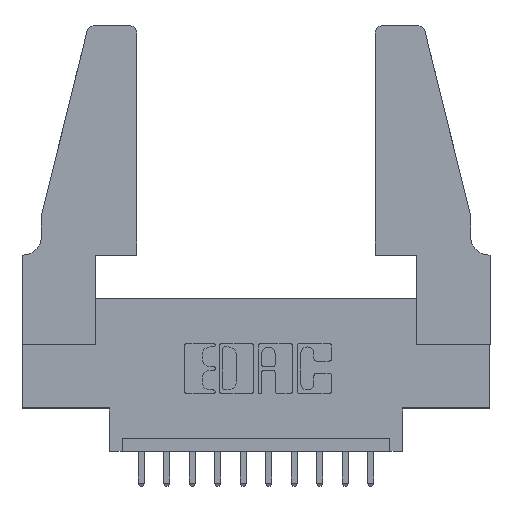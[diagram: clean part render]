
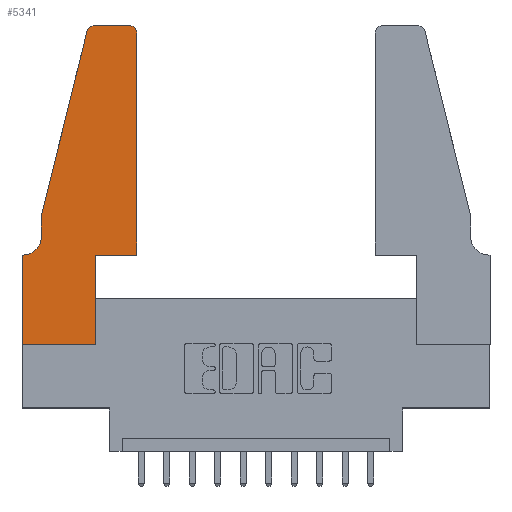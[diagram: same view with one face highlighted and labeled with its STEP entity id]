
A CAD part, top view. The second image highlights one B-rep face of the part: STEP entity #5341.
In plain terms, the highlighted planar face has unit normal (0, 0, 1).
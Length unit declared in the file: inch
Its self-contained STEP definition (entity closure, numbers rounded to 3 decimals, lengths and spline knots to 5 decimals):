
#116 = VECTOR ( 'NONE', #14130, 39.37008 ) ;
#225 = DIRECTION ( 'NONE',  ( 1., 0., 0. ) ) ;
#244 = CARTESIAN_POINT ( 'NONE',  ( 0.0755, 0.5, 0.37 ) ) ;
#553 = LINE ( 'NONE', #610, #12202 ) ;
#570 = LINE ( 'NONE', #6288, #11690 ) ;
#610 = CARTESIAN_POINT ( 'NONE',  ( 0.0755, 0.5, 0.37 ) ) ;
#613 = LINE ( 'NONE', #7789, #11924 ) ;
#923 = ORIENTED_EDGE ( 'NONE', *, *, #2108, .T. ) ;
#1114 = LINE ( 'NONE', #244, #11222 ) ;
#1170 = EDGE_CURVE ( 'NONE', #7994, #9981, #3850, .T. ) ;
#1179 = DIRECTION ( 'NONE',  ( 0., -1., 0. ) ) ;
#1343 = CARTESIAN_POINT ( 'NONE',  ( 0.2865, 0., 0.37 ) ) ;
#1762 = EDGE_CURVE ( 'NONE', #8534, #10032, #3019, .T. ) ;
#1834 = VERTEX_POINT ( 'NONE', #3236 ) ;
#1952 = ORIENTED_EDGE ( 'NONE', *, *, #5141, .T. ) ;
#1980 = CARTESIAN_POINT ( 'NONE',  ( 0.0755, 0.42, 0.37 ) ) ;
#2029 = LINE ( 'NONE', #10327, #6432 ) ;
#2077 = DIRECTION ( 'NONE',  ( 0., 0., 1. ) ) ;
#2108 = EDGE_CURVE ( 'NONE', #8501, #3767, #1114, .T. ) ;
#2338 = VERTEX_POINT ( 'NONE', #10201 ) ;
#2632 = ORIENTED_EDGE ( 'NONE', *, *, #10831, .T. ) ;
#2747 = VERTEX_POINT ( 'NONE', #6001 ) ;
#2911 = DIRECTION ( 'NONE',  ( 1., 0., 0. ) ) ;
#3019 = LINE ( 'NONE', #13044, #116 ) ;
#3236 = CARTESIAN_POINT ( 'NONE',  ( 0.4505, 0.35, 0.37 ) ) ;
#3468 = CARTESIAN_POINT ( 'NONE',  ( 0.284, 1.22, 0.37 ) ) ;
#3531 = ORIENTED_EDGE ( 'NONE', *, *, #1170, .T. ) ;
#3741 = VERTEX_POINT ( 'NONE', #11877 ) ;
#3767 = VERTEX_POINT ( 'NONE', #1980 ) ;
#3782 = EDGE_CURVE ( 'NONE', #1834, #7994, #570, .T. ) ;
#3850 = CIRCLE ( 'NONE', #4066, 0.03 ) ;
#4029 = PLANE ( 'NONE',  #7995 ) ;
#4066 = AXIS2_PLACEMENT_3D ( 'NONE', #11871, #2077, #9725 ) ;
#4172 = DIRECTION ( 'NONE',  ( 0., 1., 0. ) ) ;
#4338 = LINE ( 'NONE', #8895, #11197 ) ;
#4553 = DIRECTION ( 'NONE',  ( 0., 0., 1. ) ) ;
#4977 = CARTESIAN_POINT ( 'NONE',  ( 0.4505, 0.35, 0.37 ) ) ;
#5032 = DIRECTION ( 'NONE',  ( 0., 0., 1. ) ) ;
#5068 = DIRECTION ( 'NONE',  ( 1., 0., 0. ) ) ;
#5141 = EDGE_CURVE ( 'NONE', #2338, #7509, #2029, .T. ) ;
#5164 = CARTESIAN_POINT ( 'NONE',  ( 0.4505, 1.22, 0.37 ) ) ;
#5341 = ADVANCED_FACE ( 'NONE', ( #8469 ), #4029, .T. ) ;
#5380 = DIRECTION ( 'NONE',  ( -1., 0., 0. ) ) ;
#5451 = ORIENTED_EDGE ( 'NONE', *, *, #1762, .T. ) ;
#5857 = CIRCLE ( 'NONE', #7033, 0.03 ) ;
#6001 = CARTESIAN_POINT ( 'NONE',  ( 0.284, 1.25, 0.37 ) ) ;
#6046 = DIRECTION ( 'NONE',  ( -0.239, -0.971, 0. ) ) ;
#6053 = LINE ( 'NONE', #12047, #7571 ) ;
#6288 = CARTESIAN_POINT ( 'NONE',  ( 0.4505, 0.35, 0.37 ) ) ;
#6432 = VECTOR ( 'NONE', #8199, 39.37008 ) ;
#6453 = VECTOR ( 'NONE', #5068, 39.37008 ) ;
#6905 = EDGE_CURVE ( 'NONE', #9981, #2747, #6053, .T. ) ;
#6996 = VERTEX_POINT ( 'NONE', #13892 ) ;
#7033 = AXIS2_PLACEMENT_3D ( 'NONE', #3468, #4553, #225 ) ;
#7396 = CIRCLE ( 'NONE', #14158, 0.07 ) ;
#7486 = DIRECTION ( 'NONE',  ( -1., 0., 0. ) ) ;
#7509 = VERTEX_POINT ( 'NONE', #8205 ) ;
#7548 = EDGE_LOOP ( 'NONE', ( #11158, #7769, #9499, #923, #12934, #1952, #10941, #5451, #8616, #2632, #12844, #3531 ) ) ;
#7571 = VECTOR ( 'NONE', #5380, 39.37008 ) ;
#7769 = ORIENTED_EDGE ( 'NONE', *, *, #7992, .T. ) ;
#7789 = CARTESIAN_POINT ( 'NONE',  ( 0.2865, 0.35, 0.37 ) ) ;
#7860 = EDGE_CURVE ( 'NONE', #10032, #6996, #613, .T. ) ;
#7992 = EDGE_CURVE ( 'NONE', #2747, #3741, #5857, .T. ) ;
#7994 = VERTEX_POINT ( 'NONE', #5164 ) ;
#7995 = AXIS2_PLACEMENT_3D ( 'NONE', #11620, #5032, #2911 ) ;
#8199 = DIRECTION ( 'NONE',  ( -1., 0., 0. ) ) ;
#8205 = CARTESIAN_POINT ( 'NONE',  ( 0., 0.35, 0.37 ) ) ;
#8469 = FACE_OUTER_BOUND ( 'NONE', #7548, .T. ) ;
#8501 = VERTEX_POINT ( 'NONE', #12493 ) ;
#8534 = VERTEX_POINT ( 'NONE', #11378 ) ;
#8616 = ORIENTED_EDGE ( 'NONE', *, *, #7860, .T. ) ;
#8895 = CARTESIAN_POINT ( 'NONE',  ( 0., 0., 0.37 ) ) ;
#8913 = DIRECTION ( 'NONE',  ( 0., 1., 0. ) ) ;
#9499 = ORIENTED_EDGE ( 'NONE', *, *, #13768, .T. ) ;
#9725 = DIRECTION ( 'NONE',  ( 1., 0., 0. ) ) ;
#9981 = VERTEX_POINT ( 'NONE', #13862 ) ;
#10002 = CARTESIAN_POINT ( 'NONE',  ( 0.0055, 0.42, 0.37 ) ) ;
#10032 = VERTEX_POINT ( 'NONE', #1343 ) ;
#10045 = DIRECTION ( 'NONE',  ( 0., -1., 0. ) ) ;
#10201 = CARTESIAN_POINT ( 'NONE',  ( 0.0055, 0.35, 0.37 ) ) ;
#10327 = CARTESIAN_POINT ( 'NONE',  ( 0.0755, 0.35, 0.37 ) ) ;
#10831 = EDGE_CURVE ( 'NONE', #6996, #1834, #12508, .T. ) ;
#10941 = ORIENTED_EDGE ( 'NONE', *, *, #12153, .T. ) ;
#11106 = DIRECTION ( 'NONE',  ( 0., 0., -1. ) ) ;
#11158 = ORIENTED_EDGE ( 'NONE', *, *, #6905, .T. ) ;
#11197 = VECTOR ( 'NONE', #10045, 39.37008 ) ;
#11222 = VECTOR ( 'NONE', #1179, 39.37008 ) ;
#11239 = EDGE_CURVE ( 'NONE', #3767, #2338, #7396, .T. ) ;
#11378 = CARTESIAN_POINT ( 'NONE',  ( 0., 0., 0.37 ) ) ;
#11620 = CARTESIAN_POINT ( 'NONE',  ( 0., 0.35, 0.37 ) ) ;
#11690 = VECTOR ( 'NONE', #4172, 39.37008 ) ;
#11871 = CARTESIAN_POINT ( 'NONE',  ( 0.4205, 1.22, 0.37 ) ) ;
#11877 = CARTESIAN_POINT ( 'NONE',  ( 0.25487, 1.22718, 0.37 ) ) ;
#11924 = VECTOR ( 'NONE', #8913, 39.37008 ) ;
#12047 = CARTESIAN_POINT ( 'NONE',  ( 0.2605, 1.25, 0.37 ) ) ;
#12153 = EDGE_CURVE ( 'NONE', #7509, #8534, #4338, .T. ) ;
#12202 = VECTOR ( 'NONE', #6046, 39.37008 ) ;
#12493 = CARTESIAN_POINT ( 'NONE',  ( 0.0755, 0.5, 0.37 ) ) ;
#12508 = LINE ( 'NONE', #4977, #6453 ) ;
#12844 = ORIENTED_EDGE ( 'NONE', *, *, #3782, .T. ) ;
#12934 = ORIENTED_EDGE ( 'NONE', *, *, #11239, .T. ) ;
#13044 = CARTESIAN_POINT ( 'NONE',  ( 0., 0., 0.37 ) ) ;
#13768 = EDGE_CURVE ( 'NONE', #3741, #8501, #553, .T. ) ;
#13862 = CARTESIAN_POINT ( 'NONE',  ( 0.4205, 1.25, 0.37 ) ) ;
#13892 = CARTESIAN_POINT ( 'NONE',  ( 0.2865, 0.35, 0.37 ) ) ;
#14130 = DIRECTION ( 'NONE',  ( 1., 0., 0. ) ) ;
#14158 = AXIS2_PLACEMENT_3D ( 'NONE', #10002, #11106, #7486 ) ;
